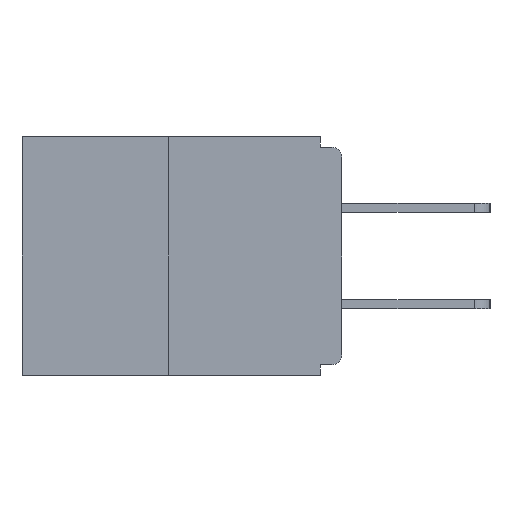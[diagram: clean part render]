
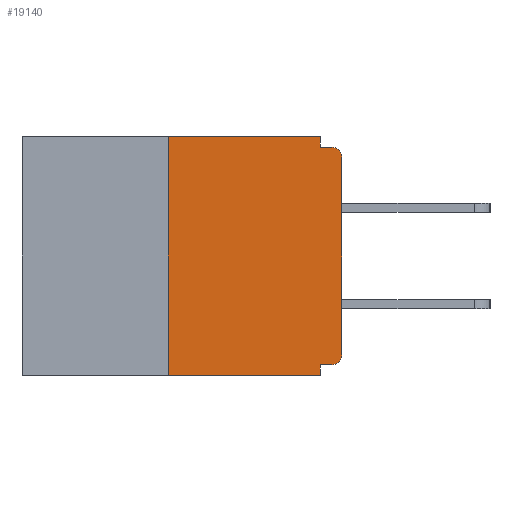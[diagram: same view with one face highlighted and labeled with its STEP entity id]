
A CAD part, left-side view. The second image highlights one B-rep face of the part: STEP entity #19140.
In plain terms, the highlighted planar face has unit normal (-1, 0, 0).
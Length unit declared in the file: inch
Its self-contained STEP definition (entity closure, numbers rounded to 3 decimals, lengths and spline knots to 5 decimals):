
#125 = DIRECTION ( 'NONE',  ( 0., 0., 1. ) ) ;
#294 = CARTESIAN_POINT ( 'NONE',  ( 0., 0.031, -0.328 ) ) ;
#308 = VERTEX_POINT ( 'NONE', #20687 ) ;
#903 = PLANE ( 'NONE',  #1865 ) ;
#936 = VERTEX_POINT ( 'NONE', #294 ) ;
#1170 = VECTOR ( 'NONE', #22739, 39.37008 ) ;
#1213 = CARTESIAN_POINT ( 'NONE',  ( 0., 0.031, -0.015 ) ) ;
#1272 = EDGE_CURVE ( 'NONE', #18203, #6659, #16363, .T. ) ;
#1840 = LINE ( 'NONE', #16386, #1170 ) ;
#1865 = AXIS2_PLACEMENT_3D ( 'NONE', #13888, #16026, #13529 ) ;
#1987 = EDGE_CURVE ( 'NONE', #308, #8287, #1840, .T. ) ;
#2018 = FACE_OUTER_BOUND ( 'NONE', #27282, .T. ) ;
#2100 = CIRCLE ( 'NONE', #15390, 0.015 ) ;
#3119 = VECTOR ( 'NONE', #24735, 39.37008 ) ;
#3325 = CARTESIAN_POINT ( 'NONE',  ( 0., 0.031, -0.343 ) ) ;
#3363 = VERTEX_POINT ( 'NONE', #6597 ) ;
#3540 = EDGE_CURVE ( 'NONE', #17815, #18203, #22952, .T. ) ;
#3650 = CARTESIAN_POINT ( 'NONE',  ( 0., 0., -0.015 ) ) ;
#3793 = VERTEX_POINT ( 'NONE', #24992 ) ;
#4706 = VERTEX_POINT ( 'NONE', #7787 ) ;
#5491 = ORIENTED_EDGE ( 'NONE', *, *, #11642, .F. ) ;
#5649 = ORIENTED_EDGE ( 'NONE', *, *, #1987, .F. ) ;
#6597 = CARTESIAN_POINT ( 'NONE',  ( 0., 0.031, -0.343 ) ) ;
#6659 = VERTEX_POINT ( 'NONE', #19379 ) ;
#6713 = LINE ( 'NONE', #18298, #26953 ) ;
#6787 = ORIENTED_EDGE ( 'NONE', *, *, #22995, .T. ) ;
#7068 = CARTESIAN_POINT ( 'NONE',  ( 0., 0.015, -0.313 ) ) ;
#7114 = CARTESIAN_POINT ( 'NONE',  ( 0., 0.015, -0.03 ) ) ;
#7135 = ORIENTED_EDGE ( 'NONE', *, *, #20281, .F. ) ;
#7787 = CARTESIAN_POINT ( 'NONE',  ( 0., 0., -0.03 ) ) ;
#7943 = VECTOR ( 'NONE', #20203, 39.37008 ) ;
#8220 = LINE ( 'NONE', #27513, #15184 ) ;
#8287 = VERTEX_POINT ( 'NONE', #14595 ) ;
#8696 = AXIS2_PLACEMENT_3D ( 'NONE', #7114, #13689, #9320 ) ;
#9320 = DIRECTION ( 'NONE',  ( 0., 0., -1. ) ) ;
#10049 = DIRECTION ( 'NONE',  ( 0., -1., 0. ) ) ;
#10225 = VECTOR ( 'NONE', #23602, 39.37008 ) ;
#11642 = EDGE_CURVE ( 'NONE', #26135, #936, #6713, .T. ) ;
#12306 = ORIENTED_EDGE ( 'NONE', *, *, #13849, .T. ) ;
#12448 = ORIENTED_EDGE ( 'NONE', *, *, #1272, .F. ) ;
#12859 = LINE ( 'NONE', #24778, #20450 ) ;
#13218 = EDGE_CURVE ( 'NONE', #4706, #6659, #16543, .T. ) ;
#13529 = DIRECTION ( 'NONE',  ( 0., 0., -1. ) ) ;
#13689 = DIRECTION ( 'NONE',  ( -1., 0., 0. ) ) ;
#13849 = EDGE_CURVE ( 'NONE', #3793, #4706, #8220, .T. ) ;
#13888 = CARTESIAN_POINT ( 'NONE',  ( 0., 0.46, 0. ) ) ;
#13923 = LINE ( 'NONE', #3325, #7943 ) ;
#14595 = CARTESIAN_POINT ( 'NONE',  ( 0., 0.25, 0. ) ) ;
#15184 = VECTOR ( 'NONE', #125, 39.37008 ) ;
#15390 = AXIS2_PLACEMENT_3D ( 'NONE', #7068, #26167, #25792 ) ;
#16026 = DIRECTION ( 'NONE',  ( 1., 0., 0. ) ) ;
#16078 = DIRECTION ( 'NONE',  ( 0., 1., 0. ) ) ;
#16363 = LINE ( 'NONE', #3650, #3119 ) ;
#16386 = CARTESIAN_POINT ( 'NONE',  ( 0., 0.25, 0. ) ) ;
#16543 = CIRCLE ( 'NONE', #8696, 0.015 ) ;
#16946 = CARTESIAN_POINT ( 'NONE',  ( 0., 0.46, -0.343 ) ) ;
#17815 = VERTEX_POINT ( 'NONE', #25516 ) ;
#17889 = LINE ( 'NONE', #16946, #10225 ) ;
#18203 = VERTEX_POINT ( 'NONE', #1213 ) ;
#18298 = CARTESIAN_POINT ( 'NONE',  ( 0., 0., -0.328 ) ) ;
#18528 = ORIENTED_EDGE ( 'NONE', *, *, #3540, .F. ) ;
#19140 = ADVANCED_FACE ( 'NONE', ( #2018 ), #903, .F. ) ;
#19379 = CARTESIAN_POINT ( 'NONE',  ( 0., 0.015, -0.015 ) ) ;
#19446 = ORIENTED_EDGE ( 'NONE', *, *, #20731, .T. ) ;
#19529 = CARTESIAN_POINT ( 'NONE',  ( 0., 0.031, 0. ) ) ;
#19799 = DIRECTION ( 'NONE',  ( 0., 0., -1. ) ) ;
#20203 = DIRECTION ( 'NONE',  ( 0., 0., -1. ) ) ;
#20281 = EDGE_CURVE ( 'NONE', #936, #3363, #13923, .T. ) ;
#20450 = VECTOR ( 'NONE', #10049, 39.37008 ) ;
#20687 = CARTESIAN_POINT ( 'NONE',  ( 0., 0.25, -0.343 ) ) ;
#20731 = EDGE_CURVE ( 'NONE', #26135, #3793, #2100, .T. ) ;
#22739 = DIRECTION ( 'NONE',  ( 0., 0., 1. ) ) ;
#22952 = LINE ( 'NONE', #19529, #25292 ) ;
#22995 = EDGE_CURVE ( 'NONE', #308, #3363, #17889, .T. ) ;
#23352 = EDGE_CURVE ( 'NONE', #8287, #17815, #12859, .T. ) ;
#23602 = DIRECTION ( 'NONE',  ( 0., -1., 0. ) ) ;
#24735 = DIRECTION ( 'NONE',  ( 0., -1., 0. ) ) ;
#24761 = CARTESIAN_POINT ( 'NONE',  ( 0., 0.015, -0.328 ) ) ;
#24778 = CARTESIAN_POINT ( 'NONE',  ( 0., 0.46, 0. ) ) ;
#24992 = CARTESIAN_POINT ( 'NONE',  ( 0., 0., -0.313 ) ) ;
#25292 = VECTOR ( 'NONE', #19799, 39.37008 ) ;
#25516 = CARTESIAN_POINT ( 'NONE',  ( 0., 0.031, 0. ) ) ;
#25792 = DIRECTION ( 'NONE',  ( 0., 0., -1. ) ) ;
#26135 = VERTEX_POINT ( 'NONE', #24761 ) ;
#26167 = DIRECTION ( 'NONE',  ( -1., 0., 0. ) ) ;
#26184 = ORIENTED_EDGE ( 'NONE', *, *, #23352, .F. ) ;
#26294 = ORIENTED_EDGE ( 'NONE', *, *, #13218, .T. ) ;
#26953 = VECTOR ( 'NONE', #16078, 39.37008 ) ;
#27282 = EDGE_LOOP ( 'NONE', ( #26184, #5649, #6787, #7135, #5491, #19446, #12306, #26294, #12448, #18528 ) ) ;
#27513 = CARTESIAN_POINT ( 'NONE',  ( 0., 0., 0. ) ) ;
